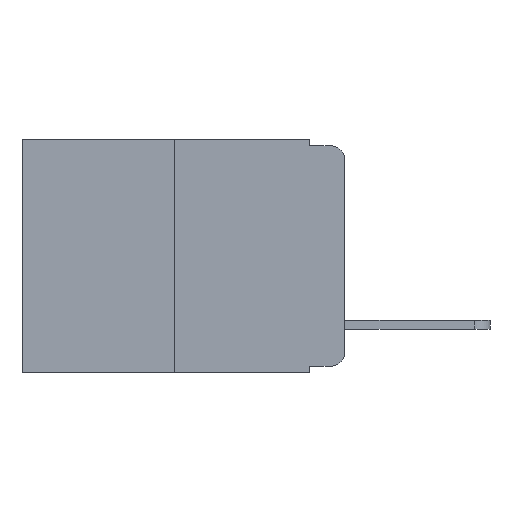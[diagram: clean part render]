
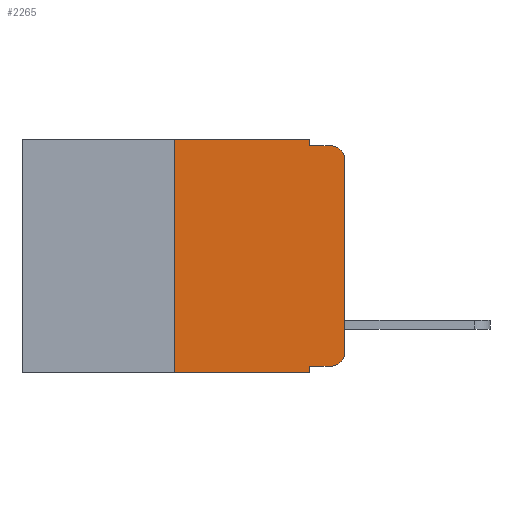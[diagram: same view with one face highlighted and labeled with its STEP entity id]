
A CAD part, left-side view. The second image highlights one B-rep face of the part: STEP entity #2265.
In plain terms, the highlighted planar face has unit normal (-1, 0, 0).
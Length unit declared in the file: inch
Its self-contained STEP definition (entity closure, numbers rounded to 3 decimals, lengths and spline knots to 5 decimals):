
#331 = CARTESIAN_POINT ( 'NONE',  ( 0., 0.25, -0.343 ) ) ;
#536 = VECTOR ( 'NONE', #8674, 39.37008 ) ;
#556 = CARTESIAN_POINT ( 'NONE',  ( 0., 0.051, -0.333 ) ) ;
#570 = LINE ( 'NONE', #8740, #536 ) ;
#596 = VECTOR ( 'NONE', #5559, 39.37008 ) ;
#662 = LINE ( 'NONE', #6648, #596 ) ;
#715 = CARTESIAN_POINT ( 'NONE',  ( 0., 0.051, -0.343 ) ) ;
#848 = VERTEX_POINT ( 'NONE', #2572 ) ;
#889 = VECTOR ( 'NONE', #8164, 39.37008 ) ;
#1036 = CARTESIAN_POINT ( 'NONE',  ( 0., 0.051, -0.01 ) ) ;
#1099 = LINE ( 'NONE', #3041, #889 ) ;
#1114 = VERTEX_POINT ( 'NONE', #556 ) ;
#1291 = VECTOR ( 'NONE', #10588, 39.37008 ) ;
#1338 = LINE ( 'NONE', #6868, #1291 ) ;
#1550 = EDGE_CURVE ( 'NONE', #2364, #5210, #4354, .T. ) ;
#1609 = EDGE_LOOP ( 'NONE', ( #9251, #11226, #3673, #5674, #7992, #9683, #12029, #3110, #3652, #3886 ) ) ;
#1836 = VECTOR ( 'NONE', #2601, 39.37008 ) ;
#1888 = DIRECTION ( 'NONE',  ( 0., -1., 0. ) ) ;
#1920 = CARTESIAN_POINT ( 'NONE',  ( 0., 0.473, 0. ) ) ;
#2036 = LINE ( 'NONE', #1036, #1836 ) ;
#2055 = CIRCLE ( 'NONE', #10484, 0.02 ) ;
#2250 = VECTOR ( 'NONE', #4197, 39.37008 ) ;
#2265 = ADVANCED_FACE ( 'NONE', ( #10704 ), #10640, .F. ) ;
#2285 = LINE ( 'NONE', #5779, #2250 ) ;
#2364 = VERTEX_POINT ( 'NONE', #331 ) ;
#2572 = CARTESIAN_POINT ( 'NONE',  ( 0., 0.02, -0.01 ) ) ;
#2601 = DIRECTION ( 'NONE',  ( 0., -1., 0. ) ) ;
#2618 = DIRECTION ( 'NONE',  ( 0., 0., -1. ) ) ;
#3041 = CARTESIAN_POINT ( 'NONE',  ( 0., 0.25, 0. ) ) ;
#3110 = ORIENTED_EDGE ( 'NONE', *, *, #3584, .F. ) ;
#3327 = EDGE_CURVE ( 'NONE', #12324, #7903, #2285, .T. ) ;
#3382 = EDGE_CURVE ( 'NONE', #7903, #848, #2055, .T. ) ;
#3405 = EDGE_CURVE ( 'NONE', #3707, #848, #2036, .T. ) ;
#3474 = EDGE_CURVE ( 'NONE', #5618, #3707, #1338, .T. ) ;
#3497 = EDGE_CURVE ( 'NONE', #2364, #10702, #1099, .T. ) ;
#3584 = EDGE_CURVE ( 'NONE', #1114, #5210, #570, .T. ) ;
#3605 = EDGE_CURVE ( 'NONE', #1114, #5490, #662, .T. ) ;
#3652 = ORIENTED_EDGE ( 'NONE', *, *, #3605, .T. ) ;
#3673 = ORIENTED_EDGE ( 'NONE', *, *, #3405, .F. ) ;
#3677 = EDGE_CURVE ( 'NONE', #5490, #12324, #4105, .T. ) ;
#3707 = VERTEX_POINT ( 'NONE', #9511 ) ;
#3886 = ORIENTED_EDGE ( 'NONE', *, *, #3677, .T. ) ;
#3929 = DIRECTION ( 'NONE',  ( -1., 0., 0. ) ) ;
#4105 = CIRCLE ( 'NONE', #9795, 0.02 ) ;
#4197 = DIRECTION ( 'NONE',  ( 0., 0., 1. ) ) ;
#4328 = VECTOR ( 'NONE', #8969, 39.37008 ) ;
#4354 = LINE ( 'NONE', #8733, #4328 ) ;
#5175 = DIRECTION ( 'NONE',  ( 0., 0., -1. ) ) ;
#5181 = DIRECTION ( 'NONE',  ( -1., 0., 0. ) ) ;
#5194 = CARTESIAN_POINT ( 'NONE',  ( 0., 0.02, -0.313 ) ) ;
#5210 = VERTEX_POINT ( 'NONE', #715 ) ;
#5490 = VERTEX_POINT ( 'NONE', #9746 ) ;
#5559 = DIRECTION ( 'NONE',  ( 0., -1., 0. ) ) ;
#5618 = VERTEX_POINT ( 'NONE', #6837 ) ;
#5674 = ORIENTED_EDGE ( 'NONE', *, *, #3474, .F. ) ;
#5779 = CARTESIAN_POINT ( 'NONE',  ( 0., 0., 0. ) ) ;
#6648 = CARTESIAN_POINT ( 'NONE',  ( 0., 0.051, -0.333 ) ) ;
#6824 = CARTESIAN_POINT ( 'NONE',  ( 0., 0., -0.313 ) ) ;
#6837 = CARTESIAN_POINT ( 'NONE',  ( 0., 0.051, 0. ) ) ;
#6868 = CARTESIAN_POINT ( 'NONE',  ( 0., 0.051, 0. ) ) ;
#7853 = LINE ( 'NONE', #1920, #9870 ) ;
#7903 = VERTEX_POINT ( 'NONE', #9454 ) ;
#7992 = ORIENTED_EDGE ( 'NONE', *, *, #11730, .F. ) ;
#8155 = AXIS2_PLACEMENT_3D ( 'NONE', #12006, #10596, #10557 ) ;
#8164 = DIRECTION ( 'NONE',  ( 0., 0., 1. ) ) ;
#8674 = DIRECTION ( 'NONE',  ( 0., 0., -1. ) ) ;
#8733 = CARTESIAN_POINT ( 'NONE',  ( 0., 0.473, -0.343 ) ) ;
#8740 = CARTESIAN_POINT ( 'NONE',  ( 0., 0.051, 0. ) ) ;
#8969 = DIRECTION ( 'NONE',  ( 0., -1., 0. ) ) ;
#9251 = ORIENTED_EDGE ( 'NONE', *, *, #3327, .T. ) ;
#9454 = CARTESIAN_POINT ( 'NONE',  ( 0., 0., -0.03 ) ) ;
#9511 = CARTESIAN_POINT ( 'NONE',  ( 0., 0.051, -0.01 ) ) ;
#9661 = CARTESIAN_POINT ( 'NONE',  ( 0., 0.25, 0. ) ) ;
#9683 = ORIENTED_EDGE ( 'NONE', *, *, #3497, .F. ) ;
#9746 = CARTESIAN_POINT ( 'NONE',  ( 0., 0.02, -0.333 ) ) ;
#9795 = AXIS2_PLACEMENT_3D ( 'NONE', #5194, #5181, #5175 ) ;
#9825 = CARTESIAN_POINT ( 'NONE',  ( 0., 0.02, -0.03 ) ) ;
#9870 = VECTOR ( 'NONE', #1888, 39.37008 ) ;
#10484 = AXIS2_PLACEMENT_3D ( 'NONE', #9825, #3929, #2618 ) ;
#10557 = DIRECTION ( 'NONE',  ( 0., 0., -1. ) ) ;
#10588 = DIRECTION ( 'NONE',  ( 0., 0., -1. ) ) ;
#10596 = DIRECTION ( 'NONE',  ( 1., 0., 0. ) ) ;
#10640 = PLANE ( 'NONE',  #8155 ) ;
#10702 = VERTEX_POINT ( 'NONE', #9661 ) ;
#10704 = FACE_OUTER_BOUND ( 'NONE', #1609, .T. ) ;
#11226 = ORIENTED_EDGE ( 'NONE', *, *, #3382, .T. ) ;
#11730 = EDGE_CURVE ( 'NONE', #10702, #5618, #7853, .T. ) ;
#12006 = CARTESIAN_POINT ( 'NONE',  ( 0., 0.473, 0. ) ) ;
#12029 = ORIENTED_EDGE ( 'NONE', *, *, #1550, .T. ) ;
#12324 = VERTEX_POINT ( 'NONE', #6824 ) ;
